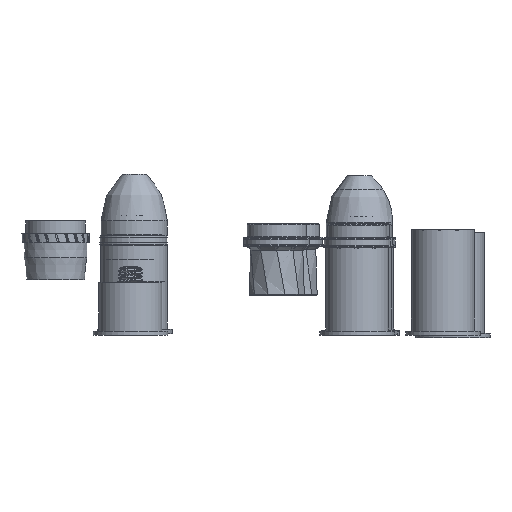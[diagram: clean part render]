
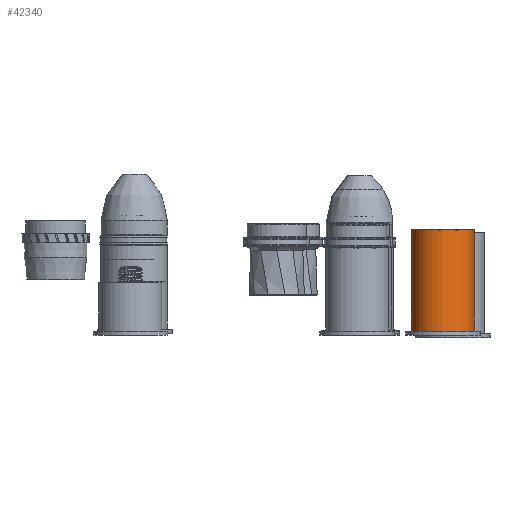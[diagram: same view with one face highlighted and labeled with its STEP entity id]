
A CAD part, left-side view. The second image highlights one B-rep face of the part: STEP entity #42340.
In plain terms, the highlighted cylindrical face has radius 18.05 mm (diameter 36.1 mm), a full revolution.
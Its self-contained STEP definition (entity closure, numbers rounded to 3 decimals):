
#7424=FACE_OUTER_BOUND('',#10057,.T.);
#10057=EDGE_LOOP('',(#36832,#36833,#36834,#36835));
#12842=LINE('',#154917,#15534);
#15534=VECTOR('',#49997,18.05);
#16668=CIRCLE('',#44585,18.05);
#16671=CIRCLE('',#44625,18.05);
#19882=VERTEX_POINT('',#153341);
#20027=VERTEX_POINT('',#154916);
#25586=EDGE_CURVE('',#19882,#19882,#16668,.F.);
#25802=EDGE_CURVE('',#19882,#20027,#12842,.T.);
#25803=EDGE_CURVE('',#20027,#20027,#16671,.T.);
#36832=ORIENTED_EDGE('',*,*,#25586,.F.);
#36833=ORIENTED_EDGE('',*,*,#25802,.T.);
#36834=ORIENTED_EDGE('',*,*,#25803,.F.);
#36835=ORIENTED_EDGE('',*,*,#25802,.F.);
#40366=CYLINDRICAL_SURFACE('',#44624,18.05);
#42340=ADVANCED_FACE('',(#7424),#40366,.T.);
#44585=AXIS2_PLACEMENT_3D('',#153342,#49791,#49792);
#44624=AXIS2_PLACEMENT_3D('',#154915,#49995,#49996);
#44625=AXIS2_PLACEMENT_3D('',#154918,#49998,#49999);
#49791=DIRECTION('center_axis',(0.,0.,
-1.));
#49792=DIRECTION('ref_axis',(1.,0.,0.));
#49995=DIRECTION('center_axis',(0.,0.,1.));
#49996=DIRECTION('ref_axis',(1.,0.,0.));
#49997=DIRECTION('',(0.,0.,-1.));
#49998=DIRECTION('center_axis',(0.,0.,-1.));
#49999=DIRECTION('ref_axis',(1.,0.,0.));
#153341=CARTESIAN_POINT('',(-68.05,0.,60.5));
#153342=CARTESIAN_POINT('Origin',(-50.,0.,60.5));
#154915=CARTESIAN_POINT('Origin',(-50.,0.,8.775));
#154916=CARTESIAN_POINT('',(-68.05,0.,2.5));
#154917=CARTESIAN_POINT('',(-68.05,0.,8.775));
#154918=CARTESIAN_POINT('Origin',(-50.,0.,2.5));
